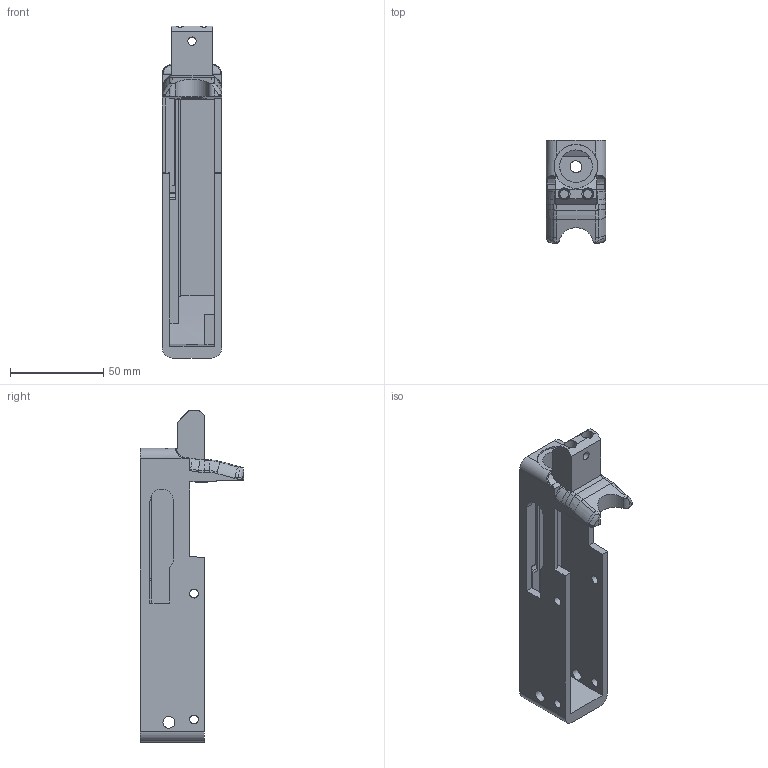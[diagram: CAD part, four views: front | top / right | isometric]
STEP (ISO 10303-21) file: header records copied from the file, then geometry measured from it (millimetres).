
FILE_DESCRIPTION(/* description */ (''),/* implementation_level */ '2;1');
FILE_NAME(/* name */ 'Ivan''FlatTop 10-22 Receiver.stp',/* time_stamp */ '2020-06-26T14:37:22-05:00',/* author */ ('johne'),/* organization */ (''),/* preprocessor_version */ 'ST-DEVELOPER v18',/* originating_system */ 'Autodesk Inventor 2020',/* authorisation */ '');
FILE_SCHEMA (('AUTOMOTIVE_DESIGN { 1 0 10303 214 3 1 1 }'));
Length unit declared in the file: inch
Products named in the file (1): receiver
Bounding box: 31.95 x 55.22 x 177.8 mm (x, y, z)
Volume: 72861.2 mm3; surface area: 35246.6 mm2
Topology: 1 solids, 2 shells, 170 faces, 477 edges, 313 vertices
Faces by surface type: plane 66, cylinder 59, bspline 40, cone 3, sphere 2
Full cylindrical faces by diameter (mm): 1.6 x1, 4.496 x1, 4.648 x2, 4.775 x4, 6.35 x3, 6.426 x2, 17.501 x1
Entity records: 6772 total; most frequent: CARTESIAN_POINT 2425, ORIENTED_EDGE 954, DIRECTION 828, EDGE_CURVE 477, VERTEX_POINT 313, AXIS2_PLACEMENT_3D 293, LINE 242, VECTOR 242
